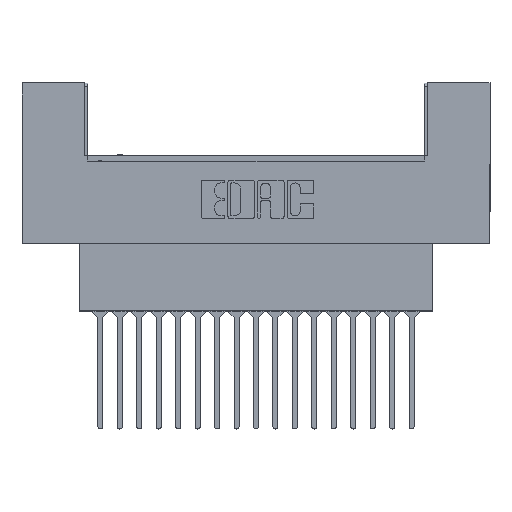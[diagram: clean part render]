
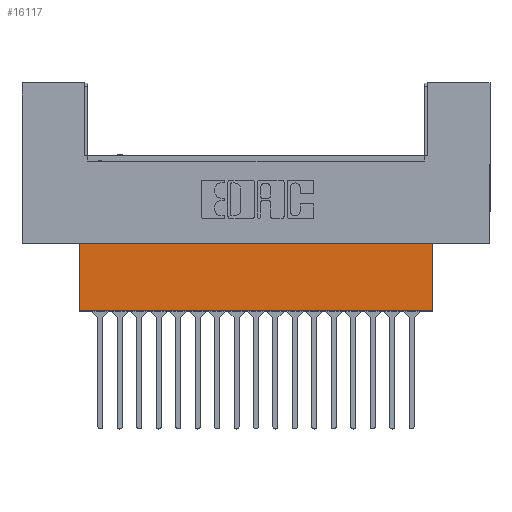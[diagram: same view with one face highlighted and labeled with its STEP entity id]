
A CAD part, top view. The second image highlights one B-rep face of the part: STEP entity #16117.
In plain terms, the highlighted planar face has unit normal (0, 0, 1).
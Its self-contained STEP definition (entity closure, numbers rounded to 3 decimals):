
#831 = VERTEX_POINT ( 'NONE', #22859 ) ;
#1104 = DIRECTION ( 'NONE',  ( -1., 0., 0. ) ) ;
#1272 = CARTESIAN_POINT ( 'NONE',  ( 53.645, -8.814, -3.962 ) ) ;
#2519 = DIRECTION ( 'NONE',  ( 0., 1., 0. ) ) ;
#2938 = CARTESIAN_POINT ( 'NONE',  ( 7.468, 0., -3.962 ) ) ;
#3435 = CARTESIAN_POINT ( 'NONE',  ( 7.468, -8.814, -3.962 ) ) ;
#4402 = AXIS2_PLACEMENT_3D ( 'NONE', #13921, #14000, #2519 ) ;
#5994 = DIRECTION ( 'NONE',  ( 0., 1., 0. ) ) ;
#6649 = CARTESIAN_POINT ( 'NONE',  ( 61.112, 0., -3.962 ) ) ;
#7174 = CARTESIAN_POINT ( 'NONE',  ( 53.645, 0., -3.962 ) ) ;
#7453 = ORIENTED_EDGE ( 'NONE', *, *, #10846, .T. ) ;
#7687 = VECTOR ( 'NONE', #14341, 1000. ) ;
#7798 = VERTEX_POINT ( 'NONE', #3435 ) ;
#8323 = DIRECTION ( 'NONE',  ( -1., 0., 0. ) ) ;
#9145 = VECTOR ( 'NONE', #1104, 1000. ) ;
#9265 = VERTEX_POINT ( 'NONE', #2938 ) ;
#10037 = VECTOR ( 'NONE', #5994, 1000. ) ;
#10583 = LINE ( 'NONE', #23230, #13539 ) ;
#10606 = LINE ( 'NONE', #20960, #10037 ) ;
#10846 = EDGE_CURVE ( 'NONE', #14222, #9265, #12067, .T. ) ;
#12067 = LINE ( 'NONE', #6649, #9145 ) ;
#12279 = ORIENTED_EDGE ( 'NONE', *, *, #22153, .F. ) ;
#13539 = VECTOR ( 'NONE', #8323, 1000. ) ;
#13579 = EDGE_LOOP ( 'NONE', ( #15952, #12279, #7453, #19985 ) ) ;
#13921 = CARTESIAN_POINT ( 'NONE',  ( 61.112, 0., -3.962 ) ) ;
#14000 = DIRECTION ( 'NONE',  ( 0., 0., -1. ) ) ;
#14222 = VERTEX_POINT ( 'NONE', #7174 ) ;
#14341 = DIRECTION ( 'NONE',  ( 0., -1., 0. ) ) ;
#14425 = EDGE_CURVE ( 'NONE', #7798, #9265, #10606, .T. ) ;
#14604 = EDGE_CURVE ( 'NONE', #831, #7798, #10583, .T. ) ;
#15952 = ORIENTED_EDGE ( 'NONE', *, *, #14604, .F. ) ;
#16117 = ADVANCED_FACE ( 'NONE', ( #22530 ), #17606, .F. ) ;
#16514 = LINE ( 'NONE', #1272, #7687 ) ;
#17606 = PLANE ( 'NONE',  #4402 ) ;
#19985 = ORIENTED_EDGE ( 'NONE', *, *, #14425, .F. ) ;
#20960 = CARTESIAN_POINT ( 'NONE',  ( 7.468, -8.814, -3.962 ) ) ;
#22153 = EDGE_CURVE ( 'NONE', #14222, #831, #16514, .T. ) ;
#22530 = FACE_OUTER_BOUND ( 'NONE', #13579, .T. ) ;
#22859 = CARTESIAN_POINT ( 'NONE',  ( 53.645, -8.814, -3.962 ) ) ;
#23230 = CARTESIAN_POINT ( 'NONE',  ( 61.112, -8.814, -3.962 ) ) ;
